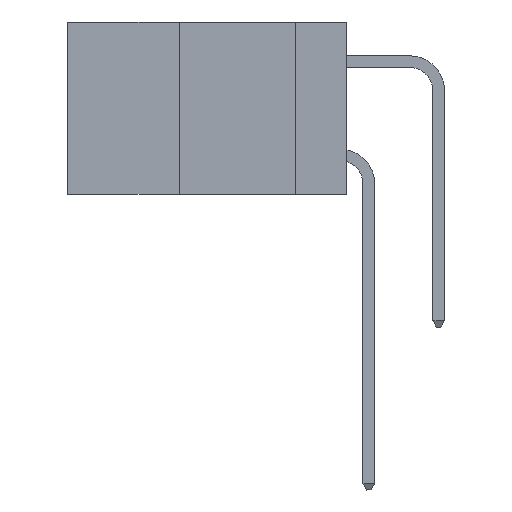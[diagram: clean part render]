
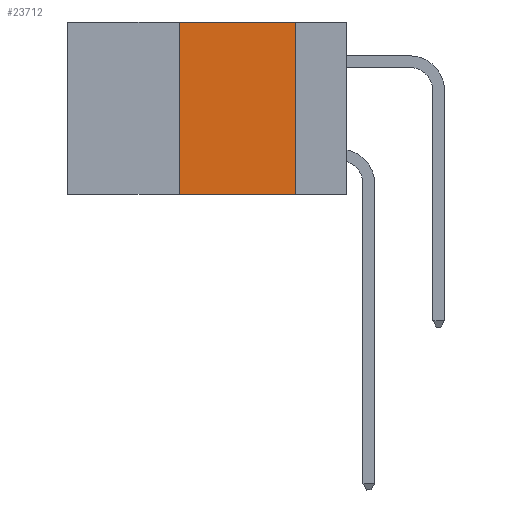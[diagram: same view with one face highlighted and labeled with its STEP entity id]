
A CAD part, left-side view. The second image highlights one B-rep face of the part: STEP entity #23712.
In plain terms, the highlighted planar face has unit normal (-1, 0, 0).
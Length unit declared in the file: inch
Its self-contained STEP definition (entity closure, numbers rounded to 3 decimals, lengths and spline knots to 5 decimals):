
#913 = ORIENTED_EDGE ( 'NONE', *, *, #25468, .T. ) ;
#2568 = EDGE_CURVE ( 'NONE', #4233, #19619, #7444, .T. ) ;
#3402 = CARTESIAN_POINT ( 'NONE',  ( 0., 0.36, 0. ) ) ;
#3676 = CARTESIAN_POINT ( 'NONE',  ( 0., 0.11, 0. ) ) ;
#4018 = CARTESIAN_POINT ( 'NONE',  ( 0., 0.36, -0.37 ) ) ;
#4233 = VERTEX_POINT ( 'NONE', #4018 ) ;
#4733 = VERTEX_POINT ( 'NONE', #3676 ) ;
#5328 = CARTESIAN_POINT ( 'NONE',  ( 0., 0.6, -0.37 ) ) ;
#5838 = CARTESIAN_POINT ( 'NONE',  ( 0., 0.6, 0. ) ) ;
#6636 = DIRECTION ( 'NONE',  ( 0., 0., -1. ) ) ;
#7444 = LINE ( 'NONE', #3402, #25072 ) ;
#8679 = EDGE_CURVE ( 'NONE', #4733, #26021, #17756, .T. ) ;
#9618 = CARTESIAN_POINT ( 'NONE',  ( 0., 0.36, 0. ) ) ;
#10225 = VECTOR ( 'NONE', #25781, 39.37008 ) ;
#10309 = CARTESIAN_POINT ( 'NONE',  ( 0., 0.11, 0. ) ) ;
#11722 = VECTOR ( 'NONE', #12028, 39.37008 ) ;
#12028 = DIRECTION ( 'NONE',  ( 0., -1., 0. ) ) ;
#15537 = PLANE ( 'NONE',  #27677 ) ;
#15669 = EDGE_LOOP ( 'NONE', ( #20179, #21537, #25643, #913 ) ) ;
#16148 = LINE ( 'NONE', #5838, #10225 ) ;
#17755 = CARTESIAN_POINT ( 'NONE',  ( 0., 0.6, 0. ) ) ;
#17756 = LINE ( 'NONE', #10309, #24229 ) ;
#19073 = DIRECTION ( 'NONE',  ( 0., 0., 1. ) ) ;
#19619 = VERTEX_POINT ( 'NONE', #9618 ) ;
#19843 = EDGE_CURVE ( 'NONE', #19619, #4733, #16148, .T. ) ;
#19960 = DIRECTION ( 'NONE',  ( 1., 0., 0. ) ) ;
#20179 = ORIENTED_EDGE ( 'NONE', *, *, #8679, .F. ) ;
#20473 = CARTESIAN_POINT ( 'NONE',  ( 0., 0.11, -0.37 ) ) ;
#21537 = ORIENTED_EDGE ( 'NONE', *, *, #19843, .F. ) ;
#22731 = LINE ( 'NONE', #5328, #11722 ) ;
#23509 = FACE_OUTER_BOUND ( 'NONE', #15669, .T. ) ;
#23712 = ADVANCED_FACE ( 'NONE', ( #23509 ), #15537, .F. ) ;
#24229 = VECTOR ( 'NONE', #27887, 39.37008 ) ;
#25072 = VECTOR ( 'NONE', #19073, 39.37008 ) ;
#25468 = EDGE_CURVE ( 'NONE', #4233, #26021, #22731, .T. ) ;
#25643 = ORIENTED_EDGE ( 'NONE', *, *, #2568, .F. ) ;
#25781 = DIRECTION ( 'NONE',  ( 0., -1., 0. ) ) ;
#26021 = VERTEX_POINT ( 'NONE', #20473 ) ;
#27677 = AXIS2_PLACEMENT_3D ( 'NONE', #17755, #19960, #6636 ) ;
#27887 = DIRECTION ( 'NONE',  ( 0., 0., -1. ) ) ;
